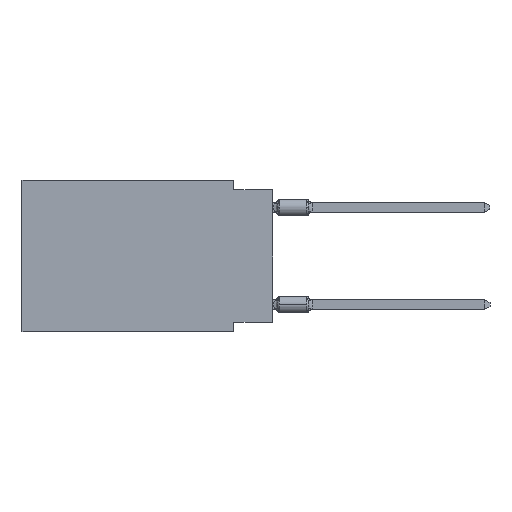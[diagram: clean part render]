
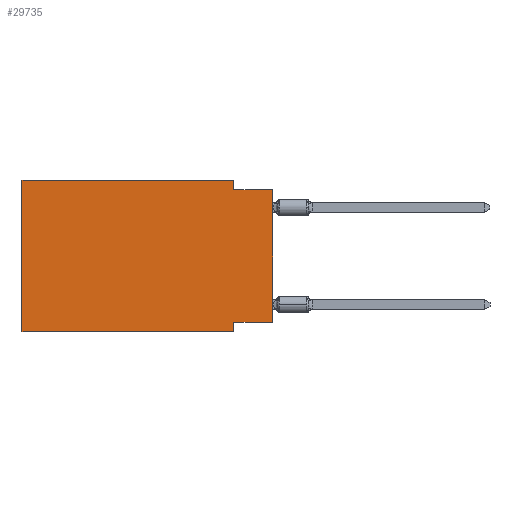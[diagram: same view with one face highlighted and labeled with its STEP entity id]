
A CAD part, left-side view. The second image highlights one B-rep face of the part: STEP entity #29735.
In plain terms, the highlighted planar face has unit normal (-1, 0, 0).
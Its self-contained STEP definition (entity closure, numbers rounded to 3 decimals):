
#60 = ORIENTED_EDGE ( 'NONE', *, *, #19210, .T. ) ;
#434 = DIRECTION ( 'NONE',  ( 0., 0., 1. ) ) ;
#1008 = LINE ( 'NONE', #27327, #32820 ) ;
#1990 = EDGE_CURVE ( 'NONE', #14648, #29911, #21129, .T. ) ;
#3778 = DIRECTION ( 'NONE',  ( 0., 0., 1. ) ) ;
#3909 = LINE ( 'NONE', #14376, #24296 ) ;
#3942 = LINE ( 'NONE', #9091, #21908 ) ;
#4138 = PLANE ( 'NONE',  #32654 ) ;
#4278 = LINE ( 'NONE', #25257, #14029 ) ;
#4967 = DIRECTION ( 'NONE',  ( 0., -1., 0. ) ) ;
#5649 = DIRECTION ( 'NONE',  ( 0., -1., 0. ) ) ;
#7343 = VECTOR ( 'NONE', #434, 1000. ) ;
#8014 = CARTESIAN_POINT ( 'NONE',  ( 0., 16.383, 0. ) ) ;
#8087 = CARTESIAN_POINT ( 'NONE',  ( 0., 2.54, -9.906 ) ) ;
#8176 = CARTESIAN_POINT ( 'NONE',  ( 0., 0., -9.271 ) ) ;
#8515 = CARTESIAN_POINT ( 'NONE',  ( 0., 2.54, -9.271 ) ) ;
#8815 = CARTESIAN_POINT ( 'NONE',  ( 0., 16.383, -9.906 ) ) ;
#8835 = ORIENTED_EDGE ( 'NONE', *, *, #25745, .F. ) ;
#9091 = CARTESIAN_POINT ( 'NONE',  ( 0., 2.54, 0. ) ) ;
#9110 = EDGE_CURVE ( 'NONE', #21134, #32070, #4278, .T. ) ;
#9946 = CARTESIAN_POINT ( 'NONE',  ( 0., 16.383, 0. ) ) ;
#10849 = EDGE_CURVE ( 'NONE', #16043, #26694, #3909, .T. ) ;
#11041 = VERTEX_POINT ( 'NONE', #13170 ) ;
#11525 = ORIENTED_EDGE ( 'NONE', *, *, #16095, .F. ) ;
#11699 = CARTESIAN_POINT ( 'NONE',  ( 0., 16.383, 0. ) ) ;
#11754 = CARTESIAN_POINT ( 'NONE',  ( 0., 2.54, 0. ) ) ;
#12557 = ORIENTED_EDGE ( 'NONE', *, *, #15317, .T. ) ;
#12886 = CARTESIAN_POINT ( 'NONE',  ( 0., 0., -0.635 ) ) ;
#12921 = ORIENTED_EDGE ( 'NONE', *, *, #22103, .F. ) ;
#13170 = CARTESIAN_POINT ( 'NONE',  ( 0., 2.54, -9.906 ) ) ;
#14029 = VECTOR ( 'NONE', #4967, 1000. ) ;
#14376 = CARTESIAN_POINT ( 'NONE',  ( 0., 0., -9.271 ) ) ;
#14648 = VERTEX_POINT ( 'NONE', #26234 ) ;
#15317 = EDGE_CURVE ( 'NONE', #27039, #11041, #26527, .T. ) ;
#15860 = DIRECTION ( 'NONE',  ( 0., -1., 0. ) ) ;
#16043 = VERTEX_POINT ( 'NONE', #8176 ) ;
#16095 = EDGE_CURVE ( 'NONE', #27039, #21134, #18657, .T. ) ;
#18657 = LINE ( 'NONE', #8014, #7343 ) ;
#18725 = CARTESIAN_POINT ( 'NONE',  ( 0., 0., -0.635 ) ) ;
#18889 = ORIENTED_EDGE ( 'NONE', *, *, #10849, .F. ) ;
#19210 = EDGE_CURVE ( 'NONE', #16043, #29911, #1008, .T. ) ;
#19215 = VECTOR ( 'NONE', #5649, 1000. ) ;
#19770 = FACE_OUTER_BOUND ( 'NONE', #25877, .T. ) ;
#20159 = ORIENTED_EDGE ( 'NONE', *, *, #1990, .F. ) ;
#21129 = LINE ( 'NONE', #12886, #19215 ) ;
#21134 = VERTEX_POINT ( 'NONE', #9946 ) ;
#21908 = VECTOR ( 'NONE', #27328, 1000. ) ;
#22103 = EDGE_CURVE ( 'NONE', #32070, #14648, #3942, .T. ) ;
#22523 = DIRECTION ( 'NONE',  ( 1., 0., 0. ) ) ;
#22674 = VECTOR ( 'NONE', #15860, 1000. ) ;
#24296 = VECTOR ( 'NONE', #24876, 1000. ) ;
#24876 = DIRECTION ( 'NONE',  ( 0., 1., 0. ) ) ;
#25257 = CARTESIAN_POINT ( 'NONE',  ( 0., 16.383, 0. ) ) ;
#25745 = EDGE_CURVE ( 'NONE', #26694, #11041, #26148, .T. ) ;
#25877 = EDGE_LOOP ( 'NONE', ( #60, #20159, #12921, #33227, #11525, #12557, #8835, #18889 ) ) ;
#26148 = LINE ( 'NONE', #8087, #26610 ) ;
#26234 = CARTESIAN_POINT ( 'NONE',  ( 0., 2.54, -0.635 ) ) ;
#26321 = DIRECTION ( 'NONE',  ( 0., 0., -1. ) ) ;
#26527 = LINE ( 'NONE', #26700, #22674 ) ;
#26610 = VECTOR ( 'NONE', #26321, 1000. ) ;
#26694 = VERTEX_POINT ( 'NONE', #8515 ) ;
#26700 = CARTESIAN_POINT ( 'NONE',  ( 0., 16.383, -9.906 ) ) ;
#27039 = VERTEX_POINT ( 'NONE', #8815 ) ;
#27327 = CARTESIAN_POINT ( 'NONE',  ( 0., 0., 0. ) ) ;
#27328 = DIRECTION ( 'NONE',  ( 0., 0., -1. ) ) ;
#29735 = ADVANCED_FACE ( 'NONE', ( #19770 ), #4138, .F. ) ;
#29911 = VERTEX_POINT ( 'NONE', #18725 ) ;
#32070 = VERTEX_POINT ( 'NONE', #11754 ) ;
#32654 = AXIS2_PLACEMENT_3D ( 'NONE', #11699, #22523, #32667 ) ;
#32667 = DIRECTION ( 'NONE',  ( 0., 0., -1. ) ) ;
#32820 = VECTOR ( 'NONE', #3778, 1000. ) ;
#33227 = ORIENTED_EDGE ( 'NONE', *, *, #9110, .F. ) ;
